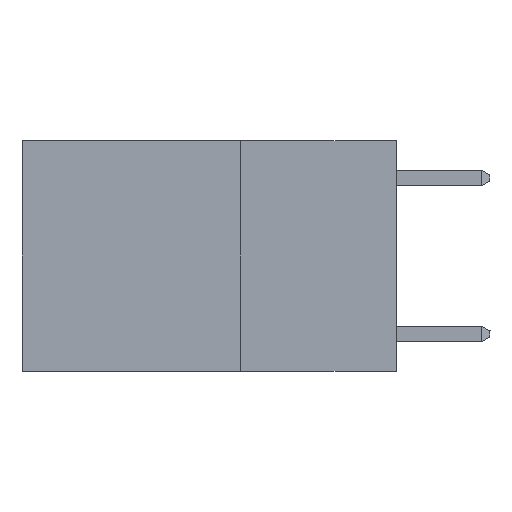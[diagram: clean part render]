
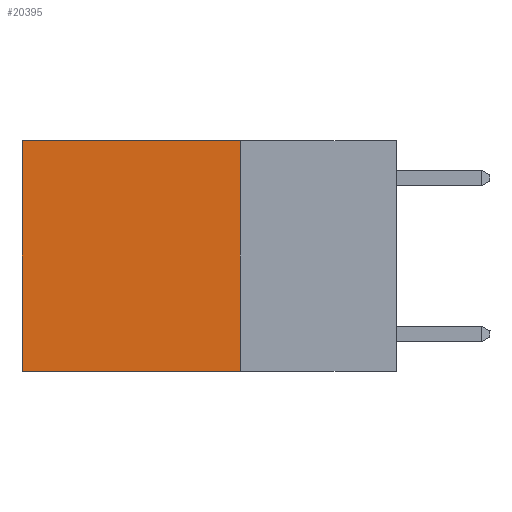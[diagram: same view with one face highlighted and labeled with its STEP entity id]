
A CAD part, left-side view. The second image highlights one B-rep face of the part: STEP entity #20395.
In plain terms, the highlighted planar face has unit normal (-1, 0, 0).
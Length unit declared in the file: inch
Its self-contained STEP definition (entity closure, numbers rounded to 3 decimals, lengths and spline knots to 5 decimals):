
#1188 = CARTESIAN_POINT ( 'NONE',  ( 0.2625, 0.25, 0. ) ) ;
#1978 = AXIS2_PLACEMENT_3D ( 'NONE', #14514, #25283, #12362 ) ;
#2311 = VECTOR ( 'NONE', #21448, 39.37008 ) ;
#2459 = FACE_OUTER_BOUND ( 'NONE', #13585, .T. ) ;
#2517 = DIRECTION ( 'NONE',  ( 0., 0., -1. ) ) ;
#3042 = EDGE_CURVE ( 'NONE', #26658, #7583, #7498, .T. ) ;
#5728 = PLANE ( 'NONE',  #1978 ) ;
#6870 = CARTESIAN_POINT ( 'NONE',  ( 0.2625, 0.25, 0. ) ) ;
#7325 = VECTOR ( 'NONE', #2517, 39.37008 ) ;
#7498 = LINE ( 'NONE', #11359, #7325 ) ;
#7550 = VECTOR ( 'NONE', #18272, 39.37008 ) ;
#7583 = VERTEX_POINT ( 'NONE', #11205 ) ;
#8459 = CARTESIAN_POINT ( 'NONE',  ( 0.2625, 0.6, 0. ) ) ;
#9882 = VERTEX_POINT ( 'NONE', #18772 ) ;
#10447 = VECTOR ( 'NONE', #20003, 39.37008 ) ;
#11045 = ORIENTED_EDGE ( 'NONE', *, *, #20712, .T. ) ;
#11205 = CARTESIAN_POINT ( 'NONE',  ( 0.2625, 0.6, -0.37 ) ) ;
#11359 = CARTESIAN_POINT ( 'NONE',  ( 0.2625, 0.6, 0. ) ) ;
#12362 = DIRECTION ( 'NONE',  ( 0., 0., -1. ) ) ;
#13585 = EDGE_LOOP ( 'NONE', ( #13880, #16304, #18558, #11045 ) ) ;
#13880 = ORIENTED_EDGE ( 'NONE', *, *, #3042, .T. ) ;
#14493 = EDGE_CURVE ( 'NONE', #9882, #7583, #19255, .T. ) ;
#14514 = CARTESIAN_POINT ( 'NONE',  ( 0.2625, 0.25, 0. ) ) ;
#16243 = EDGE_CURVE ( 'NONE', #25685, #9882, #19899, .T. ) ;
#16304 = ORIENTED_EDGE ( 'NONE', *, *, #14493, .F. ) ;
#16306 = LINE ( 'NONE', #6870, #10447 ) ;
#18272 = DIRECTION ( 'NONE',  ( 0., 1., 0. ) ) ;
#18558 = ORIENTED_EDGE ( 'NONE', *, *, #16243, .F. ) ;
#18772 = CARTESIAN_POINT ( 'NONE',  ( 0.2625, 0.25, -0.37 ) ) ;
#19255 = LINE ( 'NONE', #24476, #7550 ) ;
#19899 = LINE ( 'NONE', #25574, #2311 ) ;
#20003 = DIRECTION ( 'NONE',  ( 0., 1., 0. ) ) ;
#20395 = ADVANCED_FACE ( 'NONE', ( #2459 ), #5728, .F. ) ;
#20712 = EDGE_CURVE ( 'NONE', #25685, #26658, #16306, .T. ) ;
#21448 = DIRECTION ( 'NONE',  ( 0., 0., -1. ) ) ;
#24476 = CARTESIAN_POINT ( 'NONE',  ( 0.2625, 0.25, -0.37 ) ) ;
#25283 = DIRECTION ( 'NONE',  ( 1., 0., 0. ) ) ;
#25574 = CARTESIAN_POINT ( 'NONE',  ( 0.2625, 0.25, 0. ) ) ;
#25685 = VERTEX_POINT ( 'NONE', #1188 ) ;
#26658 = VERTEX_POINT ( 'NONE', #8459 ) ;
